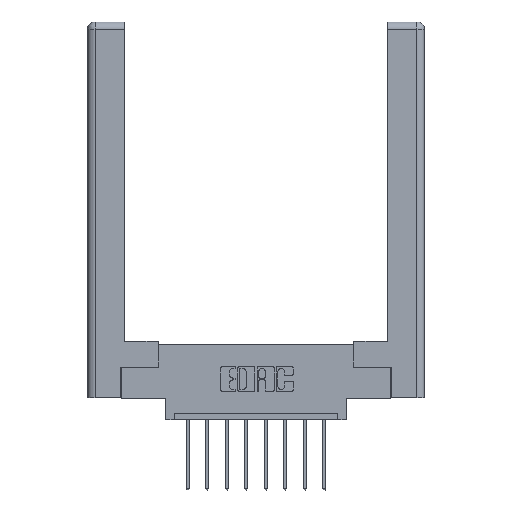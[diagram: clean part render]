
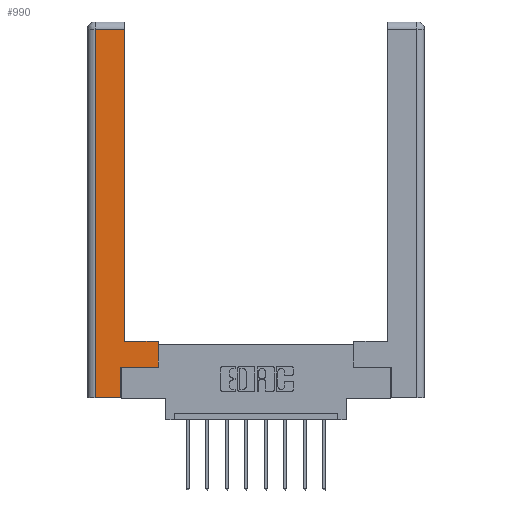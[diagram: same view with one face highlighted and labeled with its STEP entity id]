
A CAD part, top view. The second image highlights one B-rep face of the part: STEP entity #990.
In plain terms, the highlighted planar face has unit normal (0, 0, 1).
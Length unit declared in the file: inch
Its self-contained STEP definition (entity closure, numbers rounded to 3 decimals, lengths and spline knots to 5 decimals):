
#364 = PLANE ( 'NONE',  #6884 ) ;
#501 = VERTEX_POINT ( 'NONE', #4599 ) ;
#657 = DIRECTION ( 'NONE',  ( -1., 0., 0. ) ) ;
#832 = EDGE_CURVE ( 'NONE', #12474, #3463, #2225, .T. ) ;
#990 = ADVANCED_FACE ( 'NONE', ( #8235 ), #364, .F. ) ;
#1624 = ORIENTED_EDGE ( 'NONE', *, *, #11349, .T. ) ;
#1980 = CARTESIAN_POINT ( 'NONE',  ( 0.565, 0.45, 0. ) ) ;
#2073 = ORIENTED_EDGE ( 'NONE', *, *, #5363, .T. ) ;
#2225 = LINE ( 'NONE', #9956, #12202 ) ;
#2310 = LINE ( 'NONE', #9827, #7395 ) ;
#2946 = DIRECTION ( 'NONE',  ( 0., 1., 0. ) ) ;
#3095 = CARTESIAN_POINT ( 'NONE',  ( 0.565, 0.245, 0. ) ) ;
#3166 = VECTOR ( 'NONE', #2946, 39.37008 ) ;
#3198 = LINE ( 'NONE', #5456, #7636 ) ;
#3447 = VERTEX_POINT ( 'NONE', #4843 ) ;
#3463 = VERTEX_POINT ( 'NONE', #11015 ) ;
#3511 = ORIENTED_EDGE ( 'NONE', *, *, #10845, .T. ) ;
#3755 = EDGE_CURVE ( 'NONE', #3447, #7939, #7718, .T. ) ;
#3822 = EDGE_CURVE ( 'NONE', #5302, #8763, #2310, .T. ) ;
#4348 = LINE ( 'NONE', #9032, #5309 ) ;
#4599 = CARTESIAN_POINT ( 'NONE',  ( 0.295, 0.45, 0. ) ) ;
#4843 = CARTESIAN_POINT ( 'NONE',  ( 0.565, 0.245, 0. ) ) ;
#4973 = CARTESIAN_POINT ( 'NONE',  ( 0.295, 3., 0. ) ) ;
#5187 = VECTOR ( 'NONE', #10951, 39.37008 ) ;
#5302 = VERTEX_POINT ( 'NONE', #8296 ) ;
#5309 = VECTOR ( 'NONE', #6139, 39.37008 ) ;
#5329 = DIRECTION ( 'NONE',  ( -1., 0., 0. ) ) ;
#5363 = EDGE_CURVE ( 'NONE', #7939, #501, #4348, .T. ) ;
#5456 = CARTESIAN_POINT ( 'NONE',  ( 0.265, 0., 0. ) ) ;
#5667 = VERTEX_POINT ( 'NONE', #12479 ) ;
#6139 = DIRECTION ( 'NONE',  ( -1., 0., 0. ) ) ;
#6207 = DIRECTION ( 'NONE',  ( 1., 0., 0. ) ) ;
#6884 = AXIS2_PLACEMENT_3D ( 'NONE', #7362, #10393, #5329 ) ;
#6953 = ORIENTED_EDGE ( 'NONE', *, *, #7607, .T. ) ;
#7131 = LINE ( 'NONE', #3095, #9311 ) ;
#7320 = CARTESIAN_POINT ( 'NONE',  ( 0.265, 0., 0. ) ) ;
#7362 = CARTESIAN_POINT ( 'NONE',  ( 0., 0., 0. ) ) ;
#7395 = VECTOR ( 'NONE', #11871, 39.37008 ) ;
#7569 = CARTESIAN_POINT ( 'NONE',  ( 0.0615, 2.94, 0. ) ) ;
#7607 = EDGE_CURVE ( 'NONE', #501, #5667, #9641, .T. ) ;
#7636 = VECTOR ( 'NONE', #11542, 39.37008 ) ;
#7718 = LINE ( 'NONE', #1980, #5187 ) ;
#7924 = ORIENTED_EDGE ( 'NONE', *, *, #3822, .T. ) ;
#7939 = VERTEX_POINT ( 'NONE', #12812 ) ;
#8129 = EDGE_CURVE ( 'NONE', #3463, #3447, #7131, .T. ) ;
#8235 = FACE_OUTER_BOUND ( 'NONE', #9685, .T. ) ;
#8296 = CARTESIAN_POINT ( 'NONE',  ( 0.0615, 2.94, 0. ) ) ;
#8564 = ORIENTED_EDGE ( 'NONE', *, *, #3755, .T. ) ;
#8763 = VERTEX_POINT ( 'NONE', #11393 ) ;
#9032 = CARTESIAN_POINT ( 'NONE',  ( 0.295, 0.45, 0. ) ) ;
#9311 = VECTOR ( 'NONE', #6207, 39.37008 ) ;
#9574 = LINE ( 'NONE', #7569, #12936 ) ;
#9641 = LINE ( 'NONE', #4973, #3166 ) ;
#9685 = EDGE_LOOP ( 'NONE', ( #6953, #1624, #7924, #3511, #11711, #11512, #8564, #2073 ) ) ;
#9827 = CARTESIAN_POINT ( 'NONE',  ( 0.0615, 0., 0. ) ) ;
#9956 = CARTESIAN_POINT ( 'NONE',  ( 0.265, 0.245, 0. ) ) ;
#10393 = DIRECTION ( 'NONE',  ( 0., 0., -1. ) ) ;
#10845 = EDGE_CURVE ( 'NONE', #8763, #12474, #3198, .T. ) ;
#10951 = DIRECTION ( 'NONE',  ( 0., 1., 0. ) ) ;
#11015 = CARTESIAN_POINT ( 'NONE',  ( 0.265, 0.245, 0. ) ) ;
#11349 = EDGE_CURVE ( 'NONE', #5667, #5302, #9574, .T. ) ;
#11393 = CARTESIAN_POINT ( 'NONE',  ( 0.0615, 0., 0. ) ) ;
#11512 = ORIENTED_EDGE ( 'NONE', *, *, #8129, .T. ) ;
#11542 = DIRECTION ( 'NONE',  ( 1., 0., 0. ) ) ;
#11711 = ORIENTED_EDGE ( 'NONE', *, *, #832, .T. ) ;
#11871 = DIRECTION ( 'NONE',  ( 0., -1., 0. ) ) ;
#12052 = DIRECTION ( 'NONE',  ( 0., 1., 0. ) ) ;
#12202 = VECTOR ( 'NONE', #12052, 39.37008 ) ;
#12474 = VERTEX_POINT ( 'NONE', #7320 ) ;
#12479 = CARTESIAN_POINT ( 'NONE',  ( 0.295, 2.94, 0. ) ) ;
#12812 = CARTESIAN_POINT ( 'NONE',  ( 0.565, 0.45, 0. ) ) ;
#12936 = VECTOR ( 'NONE', #657, 39.37008 ) ;
